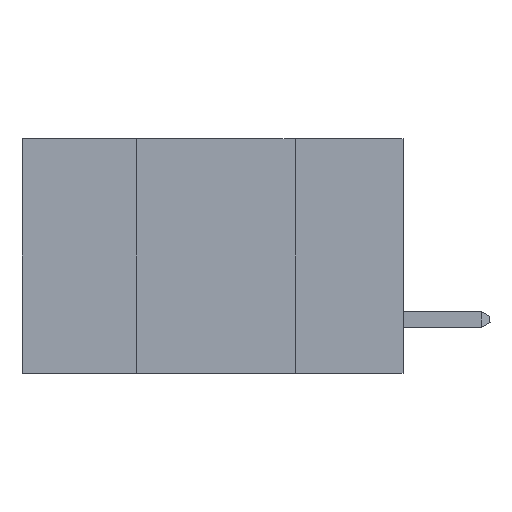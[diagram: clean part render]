
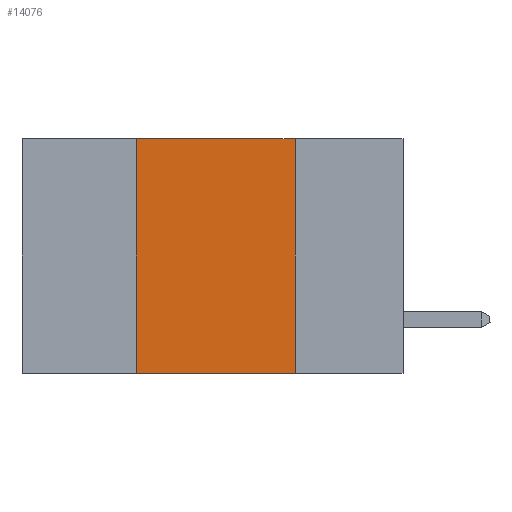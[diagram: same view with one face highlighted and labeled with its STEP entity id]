
A CAD part, left-side view. The second image highlights one B-rep face of the part: STEP entity #14076.
In plain terms, the highlighted planar face has unit normal (-1, 0, 0).
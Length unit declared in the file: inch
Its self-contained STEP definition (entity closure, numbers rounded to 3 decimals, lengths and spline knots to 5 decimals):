
#411 = VECTOR ( 'NONE', #6523, 39.37008 ) ;
#1228 = AXIS2_PLACEMENT_3D ( 'NONE', #5126, #10879, #5031 ) ;
#1312 = EDGE_CURVE ( 'NONE', #16721, #21288, #6948, .T. ) ;
#1351 = ORIENTED_EDGE ( 'NONE', *, *, #13291, .F. ) ;
#1431 = VERTEX_POINT ( 'NONE', #16659 ) ;
#2026 = ORIENTED_EDGE ( 'NONE', *, *, #1312, .F. ) ;
#3162 = DIRECTION ( 'NONE',  ( 0., 0., -1. ) ) ;
#3878 = CARTESIAN_POINT ( 'NONE',  ( 0., 0.17, 0. ) ) ;
#5031 = DIRECTION ( 'NONE',  ( 0., 0., -1. ) ) ;
#5126 = CARTESIAN_POINT ( 'NONE',  ( 0., 0.6, 0. ) ) ;
#6523 = DIRECTION ( 'NONE',  ( 0., 0., 1. ) ) ;
#6638 = DIRECTION ( 'NONE',  ( 0., -1., 0. ) ) ;
#6948 = LINE ( 'NONE', #12381, #10278 ) ;
#7432 = VECTOR ( 'NONE', #3162, 39.37008 ) ;
#7926 = ORIENTED_EDGE ( 'NONE', *, *, #8726, .T. ) ;
#8293 = VECTOR ( 'NONE', #12565, 39.37008 ) ;
#8726 = EDGE_CURVE ( 'NONE', #13863, #1431, #19388, .T. ) ;
#10278 = VECTOR ( 'NONE', #6638, 39.37008 ) ;
#10879 = DIRECTION ( 'NONE',  ( 1., 0., 0. ) ) ;
#12381 = CARTESIAN_POINT ( 'NONE',  ( 0., 0.6, 0. ) ) ;
#12565 = DIRECTION ( 'NONE',  ( 0., -1., 0. ) ) ;
#12576 = LINE ( 'NONE', #19643, #7432 ) ;
#13291 = EDGE_CURVE ( 'NONE', #21288, #1431, #12576, .T. ) ;
#13863 = VERTEX_POINT ( 'NONE', #21243 ) ;
#14076 = ADVANCED_FACE ( 'NONE', ( #18110 ), #22506, .F. ) ;
#16659 = CARTESIAN_POINT ( 'NONE',  ( 0., 0.17, -0.37 ) ) ;
#16721 = VERTEX_POINT ( 'NONE', #24873 ) ;
#18110 = FACE_OUTER_BOUND ( 'NONE', #18515, .T. ) ;
#18515 = EDGE_LOOP ( 'NONE', ( #1351, #2026, #20958, #7926 ) ) ;
#18852 = LINE ( 'NONE', #24052, #411 ) ;
#19388 = LINE ( 'NONE', #24702, #8293 ) ;
#19643 = CARTESIAN_POINT ( 'NONE',  ( 0., 0.17, 0. ) ) ;
#20958 = ORIENTED_EDGE ( 'NONE', *, *, #24378, .F. ) ;
#21243 = CARTESIAN_POINT ( 'NONE',  ( 0., 0.42, -0.37 ) ) ;
#21288 = VERTEX_POINT ( 'NONE', #3878 ) ;
#22506 = PLANE ( 'NONE',  #1228 ) ;
#24052 = CARTESIAN_POINT ( 'NONE',  ( 0., 0.42, 0. ) ) ;
#24378 = EDGE_CURVE ( 'NONE', #13863, #16721, #18852, .T. ) ;
#24702 = CARTESIAN_POINT ( 'NONE',  ( 0., 0.6, -0.37 ) ) ;
#24873 = CARTESIAN_POINT ( 'NONE',  ( 0., 0.42, 0. ) ) ;
